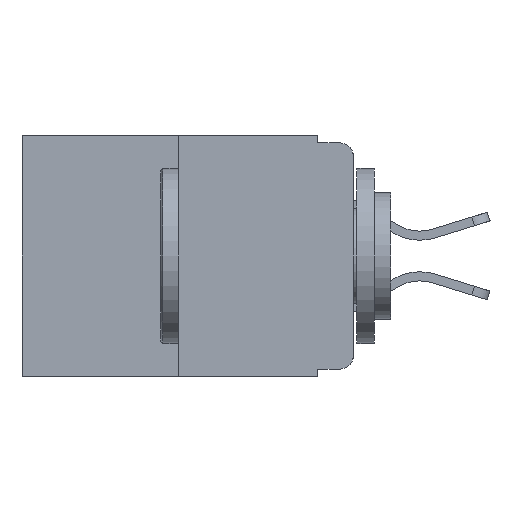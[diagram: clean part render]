
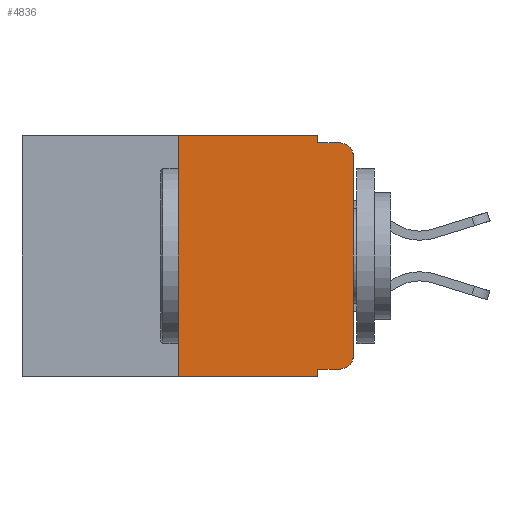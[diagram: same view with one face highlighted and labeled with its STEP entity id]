
A CAD part, left-side view. The second image highlights one B-rep face of the part: STEP entity #4836.
In plain terms, the highlighted planar face has unit normal (-1, 0, 0).
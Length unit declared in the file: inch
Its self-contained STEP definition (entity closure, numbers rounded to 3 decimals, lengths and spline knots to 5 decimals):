
#272 = LINE ( 'NONE', #10981, #19761 ) ;
#494 = VERTEX_POINT ( 'NONE', #14131 ) ;
#1251 = EDGE_LOOP ( 'NONE', ( #3174, #18775, #16142, #5003, #13214, #17957, #19702, #11482, #13235, #2947 ) ) ;
#1264 = CARTESIAN_POINT ( 'NONE',  ( 0., 0.051, -0.333 ) ) ;
#1475 = CARTESIAN_POINT ( 'NONE',  ( 0., 0.02, -0.333 ) ) ;
#1526 = DIRECTION ( 'NONE',  ( 0., -1., 0. ) ) ;
#1632 = CARTESIAN_POINT ( 'NONE',  ( 0., 0.25, -0.343 ) ) ;
#1862 = CARTESIAN_POINT ( 'NONE',  ( 0., 0.051, 0. ) ) ;
#2381 = EDGE_CURVE ( 'NONE', #6729, #22965, #21578, .T. ) ;
#2443 = DIRECTION ( 'NONE',  ( 0., -1., 0. ) ) ;
#2947 = ORIENTED_EDGE ( 'NONE', *, *, #13563, .T. ) ;
#2991 = VECTOR ( 'NONE', #3568, 39.37008 ) ;
#3104 = CARTESIAN_POINT ( 'NONE',  ( 0., 0.02, -0.313 ) ) ;
#3174 = ORIENTED_EDGE ( 'NONE', *, *, #11377, .T. ) ;
#3566 = CARTESIAN_POINT ( 'NONE',  ( 0., 0.25, 0. ) ) ;
#3568 = DIRECTION ( 'NONE',  ( 0., 0., -1. ) ) ;
#3583 = FACE_OUTER_BOUND ( 'NONE', #1251, .T. ) ;
#3927 = VECTOR ( 'NONE', #1526, 39.37008 ) ;
#4303 = EDGE_CURVE ( 'NONE', #10602, #10178, #272, .T. ) ;
#4381 = CARTESIAN_POINT ( 'NONE',  ( 0., 0.473, -0.343 ) ) ;
#4836 = ADVANCED_FACE ( 'NONE', ( #3583 ), #12671, .F. ) ;
#5003 = ORIENTED_EDGE ( 'NONE', *, *, #14355, .F. ) ;
#5029 = DIRECTION ( 'NONE',  ( 0., 0., -1. ) ) ;
#5102 = EDGE_CURVE ( 'NONE', #6431, #12088, #17109, .T. ) ;
#5198 = AXIS2_PLACEMENT_3D ( 'NONE', #19171, #7961, #21011 ) ;
#5327 = CARTESIAN_POINT ( 'NONE',  ( 0., 0.25, 0. ) ) ;
#6431 = VERTEX_POINT ( 'NONE', #17651 ) ;
#6686 = VECTOR ( 'NONE', #21303, 39.37008 ) ;
#6729 = VERTEX_POINT ( 'NONE', #3566 ) ;
#6913 = CIRCLE ( 'NONE', #20530, 0.02 ) ;
#6948 = CARTESIAN_POINT ( 'NONE',  ( 0., 0.051, -0.333 ) ) ;
#7237 = DIRECTION ( 'NONE',  ( 0., 0., 1. ) ) ;
#7363 = CARTESIAN_POINT ( 'NONE',  ( 0., 0.051, -0.343 ) ) ;
#7961 = DIRECTION ( 'NONE',  ( -1., 0., 0. ) ) ;
#8836 = DIRECTION ( 'NONE',  ( 0., -1., 0. ) ) ;
#8937 = VECTOR ( 'NONE', #8836, 39.37008 ) ;
#8953 = VERTEX_POINT ( 'NONE', #1475 ) ;
#8956 = LINE ( 'NONE', #9092, #3927 ) ;
#9092 = CARTESIAN_POINT ( 'NONE',  ( 0., 0.051, -0.01 ) ) ;
#10178 = VERTEX_POINT ( 'NONE', #7363 ) ;
#10352 = DIRECTION ( 'NONE',  ( 0., 0., -1. ) ) ;
#10602 = VERTEX_POINT ( 'NONE', #1264 ) ;
#10724 = VECTOR ( 'NONE', #13364, 39.37008 ) ;
#10808 = CARTESIAN_POINT ( 'NONE',  ( 0., 0.473, 0. ) ) ;
#10981 = CARTESIAN_POINT ( 'NONE',  ( 0., 0.051, 0. ) ) ;
#11377 = EDGE_CURVE ( 'NONE', #23732, #6431, #15723, .T. ) ;
#11482 = ORIENTED_EDGE ( 'NONE', *, *, #4303, .F. ) ;
#11830 = EDGE_CURVE ( 'NONE', #11880, #6729, #14263, .T. ) ;
#11860 = VECTOR ( 'NONE', #2443, 39.37008 ) ;
#11880 = VERTEX_POINT ( 'NONE', #1632 ) ;
#12088 = VERTEX_POINT ( 'NONE', #19265 ) ;
#12671 = PLANE ( 'NONE',  #15727 ) ;
#12794 = EDGE_CURVE ( 'NONE', #11880, #10178, #16878, .T. ) ;
#13214 = ORIENTED_EDGE ( 'NONE', *, *, #2381, .F. ) ;
#13235 = ORIENTED_EDGE ( 'NONE', *, *, #18610, .T. ) ;
#13364 = DIRECTION ( 'NONE',  ( 0., 0., 1. ) ) ;
#13563 = EDGE_CURVE ( 'NONE', #8953, #23732, #6913, .T. ) ;
#14131 = CARTESIAN_POINT ( 'NONE',  ( 0., 0.051, -0.01 ) ) ;
#14263 = LINE ( 'NONE', #5327, #23573 ) ;
#14355 = EDGE_CURVE ( 'NONE', #22965, #494, #18027, .T. ) ;
#14567 = DIRECTION ( 'NONE',  ( 0., 0., -1. ) ) ;
#15723 = LINE ( 'NONE', #22573, #10724 ) ;
#15727 = AXIS2_PLACEMENT_3D ( 'NONE', #10808, #18287, #14567 ) ;
#16076 = CARTESIAN_POINT ( 'NONE',  ( 0., 0.473, 0. ) ) ;
#16142 = ORIENTED_EDGE ( 'NONE', *, *, #18162, .F. ) ;
#16260 = DIRECTION ( 'NONE',  ( -1., 0., 0. ) ) ;
#16878 = LINE ( 'NONE', #4381, #11860 ) ;
#17109 = CIRCLE ( 'NONE', #5198, 0.02 ) ;
#17651 = CARTESIAN_POINT ( 'NONE',  ( 0., 0., -0.03 ) ) ;
#17957 = ORIENTED_EDGE ( 'NONE', *, *, #11830, .F. ) ;
#18027 = LINE ( 'NONE', #24127, #2991 ) ;
#18162 = EDGE_CURVE ( 'NONE', #494, #12088, #8956, .T. ) ;
#18287 = DIRECTION ( 'NONE',  ( 1., 0., 0. ) ) ;
#18610 = EDGE_CURVE ( 'NONE', #10602, #8953, #23775, .T. ) ;
#18775 = ORIENTED_EDGE ( 'NONE', *, *, #5102, .T. ) ;
#19171 = CARTESIAN_POINT ( 'NONE',  ( 0., 0.02, -0.03 ) ) ;
#19265 = CARTESIAN_POINT ( 'NONE',  ( 0., 0.02, -0.01 ) ) ;
#19299 = CARTESIAN_POINT ( 'NONE',  ( 0., 0., -0.313 ) ) ;
#19702 = ORIENTED_EDGE ( 'NONE', *, *, #12794, .T. ) ;
#19761 = VECTOR ( 'NONE', #10352, 39.37008 ) ;
#20530 = AXIS2_PLACEMENT_3D ( 'NONE', #3104, #16260, #5029 ) ;
#21011 = DIRECTION ( 'NONE',  ( 0., 0., -1. ) ) ;
#21303 = DIRECTION ( 'NONE',  ( 0., -1., 0. ) ) ;
#21578 = LINE ( 'NONE', #16076, #6686 ) ;
#22573 = CARTESIAN_POINT ( 'NONE',  ( 0., 0., 0. ) ) ;
#22965 = VERTEX_POINT ( 'NONE', #1862 ) ;
#23573 = VECTOR ( 'NONE', #7237, 39.37008 ) ;
#23732 = VERTEX_POINT ( 'NONE', #19299 ) ;
#23775 = LINE ( 'NONE', #6948, #8937 ) ;
#24127 = CARTESIAN_POINT ( 'NONE',  ( 0., 0.051, 0. ) ) ;
